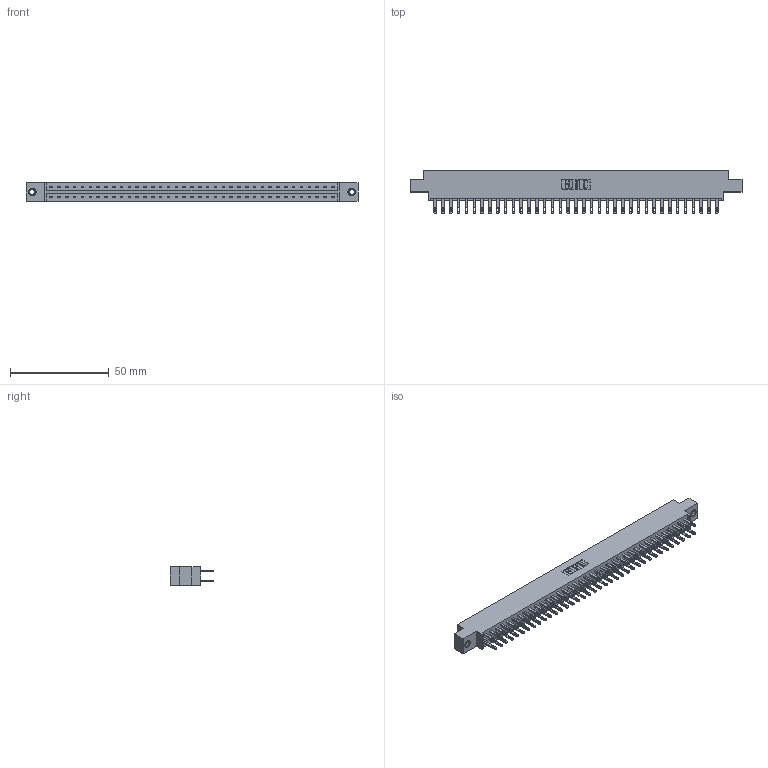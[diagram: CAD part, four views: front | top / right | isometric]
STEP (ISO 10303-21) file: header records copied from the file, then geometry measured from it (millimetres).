
FILE_DESCRIPTION (( 'STEP AP203' ), '1' );
FILE_NAME ('333-074-500-807.STEP', '2018-08-04T21:28:46', ( '' ), ( '' ), 'SwSTEP 2.0', 'SolidWorks 2016', '' );
FILE_SCHEMA (( 'CONFIG_CONTROL_DESIGN' ));
Length unit declared in the file: inch
Products named in the file (4): 333 Part_Offset - .156 Dia - TI; 345-292-001_345-293-100; 345-250-001_345-250-005-103; 333-074-500-807
Assembly tree (77 placements, depth 2):
  333-074-500-807
    333 Part_Offset - .156 Dia - TI
    345-292-001_345-293-100  x74
    345-250-001_345-250-005-103  x2
Bounding box: 168.15 x 21.85 x 9.4 mm (x, y, z)
Volume: 17105 mm3; surface area: 21237.9 mm2
Topology: 77 solids, 77 shells, 3730 faces, 11337 edges, 7550 vertices
Faces by surface type: plane 2326, cylinder 1388, cone 12, torus 4
Entity records: 25698 total; most frequent: CARTESIAN_POINT 4249, ORIENTED_EDGE 4178, DIRECTION 3671, EDGE_CURVE 2089, LINE 1937, VECTOR 1937, VERTEX_POINT 1388, AXIS2_PLACEMENT_3D 867
